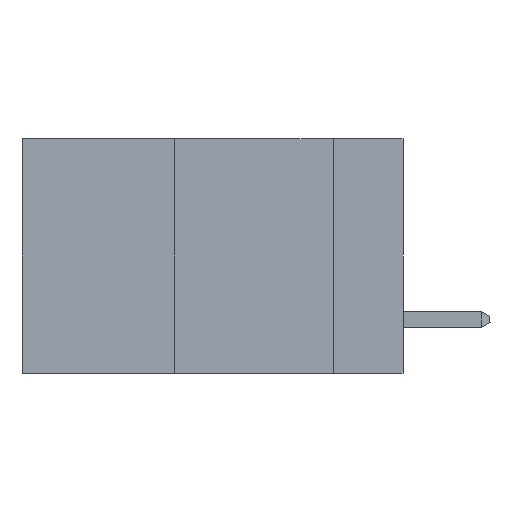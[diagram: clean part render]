
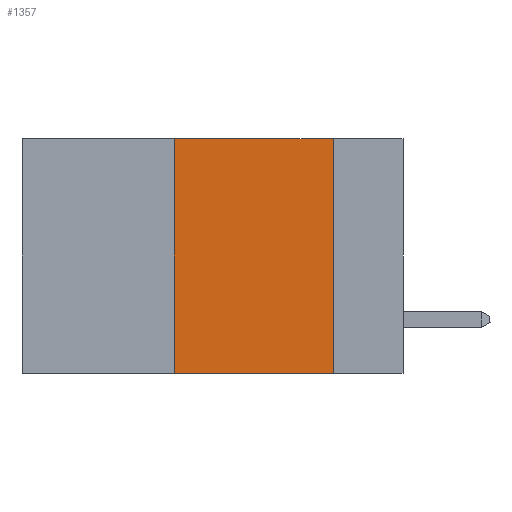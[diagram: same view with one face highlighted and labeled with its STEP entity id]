
A CAD part, left-side view. The second image highlights one B-rep face of the part: STEP entity #1357.
In plain terms, the highlighted planar face has unit normal (-1, 0, 0).
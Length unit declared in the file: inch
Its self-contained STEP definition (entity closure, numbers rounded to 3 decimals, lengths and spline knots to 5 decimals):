
#13 = VECTOR ( 'NONE', #6709, 39.37008 ) ;
#61 = AXIS2_PLACEMENT_3D ( 'NONE', #5131, #8213, #8991 ) ;
#112 = LINE ( 'NONE', #8242, #7971 ) ;
#220 = VECTOR ( 'NONE', #7808, 39.37008 ) ;
#875 = LINE ( 'NONE', #9049, #13 ) ;
#1357 = ADVANCED_FACE ( 'NONE', ( #8499 ), #9020, .F. ) ;
#1925 = CARTESIAN_POINT ( 'NONE',  ( 0., 0.36, 0. ) ) ;
#2183 = VECTOR ( 'NONE', #8771, 39.37008 ) ;
#2671 = CARTESIAN_POINT ( 'NONE',  ( 0., 0.11, 0. ) ) ;
#2713 = DIRECTION ( 'NONE',  ( 0., -1., 0. ) ) ;
#2940 = ORIENTED_EDGE ( 'NONE', *, *, #7317, .F. ) ;
#3704 = ORIENTED_EDGE ( 'NONE', *, *, #8964, .T. ) ;
#3766 = EDGE_CURVE ( 'NONE', #9690, #5680, #4271, .T. ) ;
#4271 = LINE ( 'NONE', #6382, #2183 ) ;
#5131 = CARTESIAN_POINT ( 'NONE',  ( 0., 0.6, 0. ) ) ;
#5342 = VERTEX_POINT ( 'NONE', #5836 ) ;
#5575 = EDGE_LOOP ( 'NONE', ( #9212, #9288, #2940, #3704 ) ) ;
#5680 = VERTEX_POINT ( 'NONE', #8610 ) ;
#5836 = CARTESIAN_POINT ( 'NONE',  ( 0., 0.36, -0.37 ) ) ;
#6382 = CARTESIAN_POINT ( 'NONE',  ( 0., 0.11, 0. ) ) ;
#6709 = DIRECTION ( 'NONE',  ( 0., 0., 1. ) ) ;
#7311 = VERTEX_POINT ( 'NONE', #1925 ) ;
#7317 = EDGE_CURVE ( 'NONE', #5342, #7311, #875, .T. ) ;
#7808 = DIRECTION ( 'NONE',  ( 0., -1., 0. ) ) ;
#7971 = VECTOR ( 'NONE', #2713, 39.37008 ) ;
#8213 = DIRECTION ( 'NONE',  ( 1., 0., 0. ) ) ;
#8242 = CARTESIAN_POINT ( 'NONE',  ( 0., 0.6, -0.37 ) ) ;
#8499 = FACE_OUTER_BOUND ( 'NONE', #5575, .T. ) ;
#8610 = CARTESIAN_POINT ( 'NONE',  ( 0., 0.11, -0.37 ) ) ;
#8771 = DIRECTION ( 'NONE',  ( 0., 0., -1. ) ) ;
#8964 = EDGE_CURVE ( 'NONE', #5342, #5680, #112, .T. ) ;
#8991 = DIRECTION ( 'NONE',  ( 0., 0., -1. ) ) ;
#9020 = PLANE ( 'NONE',  #61 ) ;
#9049 = CARTESIAN_POINT ( 'NONE',  ( 0., 0.36, 0. ) ) ;
#9212 = ORIENTED_EDGE ( 'NONE', *, *, #3766, .F. ) ;
#9288 = ORIENTED_EDGE ( 'NONE', *, *, #9298, .F. ) ;
#9298 = EDGE_CURVE ( 'NONE', #7311, #9690, #10141, .T. ) ;
#9397 = CARTESIAN_POINT ( 'NONE',  ( 0., 0.6, 0. ) ) ;
#9690 = VERTEX_POINT ( 'NONE', #2671 ) ;
#10141 = LINE ( 'NONE', #9397, #220 ) ;
